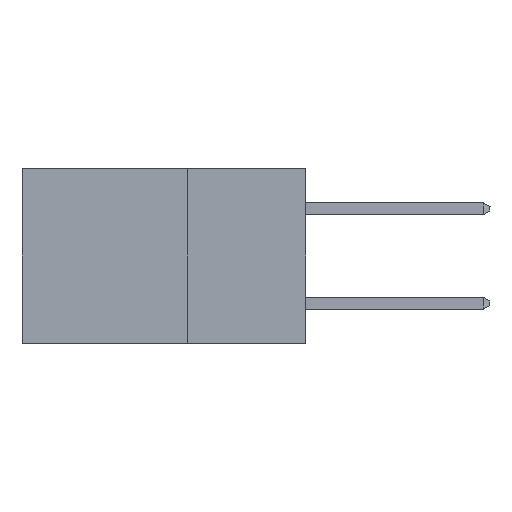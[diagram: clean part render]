
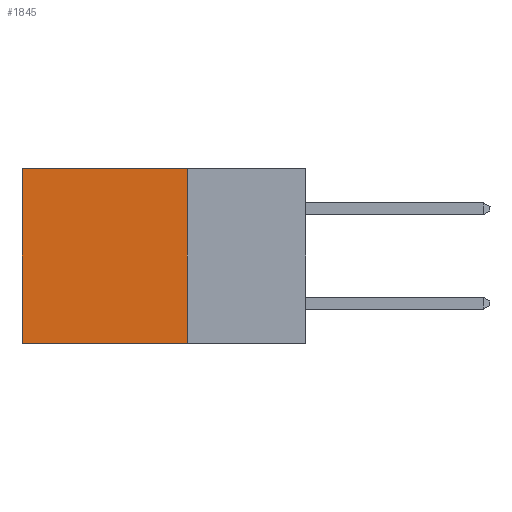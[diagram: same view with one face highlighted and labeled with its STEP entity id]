
A CAD part, left-side view. The second image highlights one B-rep face of the part: STEP entity #1845.
In plain terms, the highlighted planar face has unit normal (-1, 0, 0).
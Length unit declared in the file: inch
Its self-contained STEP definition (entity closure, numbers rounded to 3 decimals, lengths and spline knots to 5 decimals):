
#291 = VERTEX_POINT ( 'NONE', #7768 ) ;
#596 = CARTESIAN_POINT ( 'NONE',  ( 0.298, 0.25, 0. ) ) ;
#985 = LINE ( 'NONE', #9725, #13036 ) ;
#1736 = CARTESIAN_POINT ( 'NONE',  ( 0.298, 0.25, 0. ) ) ;
#1845 = ADVANCED_FACE ( 'NONE', ( #2153 ), #20863, .F. ) ;
#2153 = FACE_OUTER_BOUND ( 'NONE', #12686, .T. ) ;
#2907 = VERTEX_POINT ( 'NONE', #3407 ) ;
#3271 = AXIS2_PLACEMENT_3D ( 'NONE', #596, #11960, #5235 ) ;
#3406 = EDGE_CURVE ( 'NONE', #12272, #2907, #985, .T. ) ;
#3407 = CARTESIAN_POINT ( 'NONE',  ( 0.298, 0.6, -0.37 ) ) ;
#3483 = ORIENTED_EDGE ( 'NONE', *, *, #27826, .T. ) ;
#5109 = CARTESIAN_POINT ( 'NONE',  ( 0.298, 0.25, -0.37 ) ) ;
#5235 = DIRECTION ( 'NONE',  ( 0., 0., -1. ) ) ;
#5879 = VERTEX_POINT ( 'NONE', #27658 ) ;
#6696 = LINE ( 'NONE', #1736, #13740 ) ;
#6949 = EDGE_CURVE ( 'NONE', #5879, #12272, #27158, .T. ) ;
#7034 = ORIENTED_EDGE ( 'NONE', *, *, #3406, .F. ) ;
#7768 = CARTESIAN_POINT ( 'NONE',  ( 0.298, 0.6, 0. ) ) ;
#9038 = VECTOR ( 'NONE', #25705, 39.37008 ) ;
#9725 = CARTESIAN_POINT ( 'NONE',  ( 0.298, 0.25, -0.37 ) ) ;
#10909 = EDGE_CURVE ( 'NONE', #5879, #291, #6696, .T. ) ;
#11960 = DIRECTION ( 'NONE',  ( 1., 0., 0. ) ) ;
#12272 = VERTEX_POINT ( 'NONE', #5109 ) ;
#12686 = EDGE_LOOP ( 'NONE', ( #3483, #7034, #24726, #28234 ) ) ;
#12829 = CARTESIAN_POINT ( 'NONE',  ( 0.298, 0.6, 0. ) ) ;
#13036 = VECTOR ( 'NONE', #14360, 39.37008 ) ;
#13740 = VECTOR ( 'NONE', #15377, 39.37008 ) ;
#14360 = DIRECTION ( 'NONE',  ( 0., 1., 0. ) ) ;
#15086 = DIRECTION ( 'NONE',  ( 0., 0., -1. ) ) ;
#15377 = DIRECTION ( 'NONE',  ( 0., 1., 0. ) ) ;
#20863 = PLANE ( 'NONE',  #3271 ) ;
#21120 = CARTESIAN_POINT ( 'NONE',  ( 0.298, 0.25, 0. ) ) ;
#24726 = ORIENTED_EDGE ( 'NONE', *, *, #6949, .F. ) ;
#25435 = LINE ( 'NONE', #12829, #27253 ) ;
#25705 = DIRECTION ( 'NONE',  ( 0., 0., -1. ) ) ;
#27158 = LINE ( 'NONE', #21120, #9038 ) ;
#27253 = VECTOR ( 'NONE', #15086, 39.37008 ) ;
#27658 = CARTESIAN_POINT ( 'NONE',  ( 0.298, 0.25, 0. ) ) ;
#27826 = EDGE_CURVE ( 'NONE', #291, #2907, #25435, .T. ) ;
#28234 = ORIENTED_EDGE ( 'NONE', *, *, #10909, .T. ) ;
